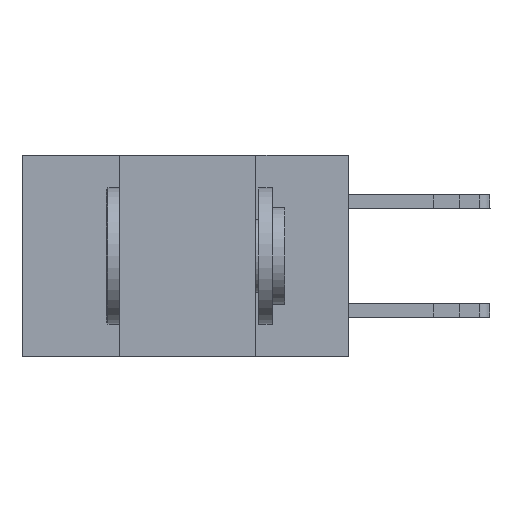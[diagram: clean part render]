
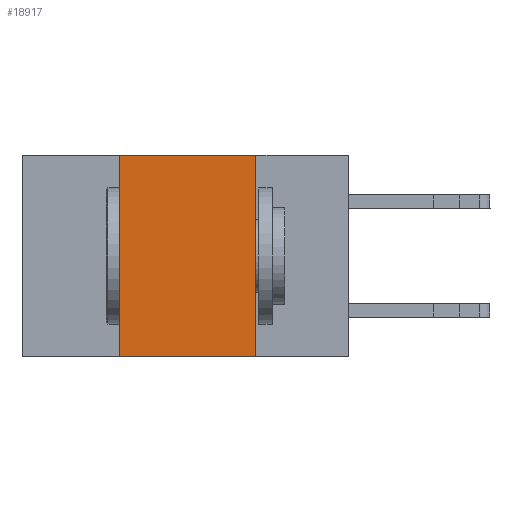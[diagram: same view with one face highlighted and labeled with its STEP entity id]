
A CAD part, left-side view. The second image highlights one B-rep face of the part: STEP entity #18917.
In plain terms, the highlighted planar face has unit normal (-1, 0, 0).
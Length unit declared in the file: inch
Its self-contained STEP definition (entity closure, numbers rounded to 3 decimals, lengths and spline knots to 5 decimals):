
#611 = VECTOR ( 'NONE', #9977, 39.37008 ) ;
#994 = CARTESIAN_POINT ( 'NONE',  ( 0., 0.6, -0.37 ) ) ;
#1306 = VERTEX_POINT ( 'NONE', #4158 ) ;
#1630 = LINE ( 'NONE', #3708, #611 ) ;
#2976 = CARTESIAN_POINT ( 'NONE',  ( 0., 0.6, 0. ) ) ;
#3246 = EDGE_CURVE ( 'NONE', #7535, #1306, #10115, .T. ) ;
#3393 = LINE ( 'NONE', #994, #19574 ) ;
#3580 = LINE ( 'NONE', #19640, #7327 ) ;
#3708 = CARTESIAN_POINT ( 'NONE',  ( 0., 0.42, 0. ) ) ;
#4158 = CARTESIAN_POINT ( 'NONE',  ( 0., 0.17, -0.37 ) ) ;
#6255 = EDGE_CURVE ( 'NONE', #6481, #7535, #3580, .T. ) ;
#6481 = VERTEX_POINT ( 'NONE', #8043 ) ;
#6937 = ORIENTED_EDGE ( 'NONE', *, *, #17049, .F. ) ;
#6992 = ORIENTED_EDGE ( 'NONE', *, *, #6255, .F. ) ;
#7317 = ORIENTED_EDGE ( 'NONE', *, *, #3246, .F. ) ;
#7327 = VECTOR ( 'NONE', #18459, 39.37008 ) ;
#7535 = VERTEX_POINT ( 'NONE', #12969 ) ;
#8043 = CARTESIAN_POINT ( 'NONE',  ( 0., 0.42, 0. ) ) ;
#8853 = VERTEX_POINT ( 'NONE', #11108 ) ;
#9977 = DIRECTION ( 'NONE',  ( 0., 0., 1. ) ) ;
#10115 = LINE ( 'NONE', #10811, #13798 ) ;
#10811 = CARTESIAN_POINT ( 'NONE',  ( 0., 0.17, 0. ) ) ;
#10896 = DIRECTION ( 'NONE',  ( 0., 0., -1. ) ) ;
#11091 = DIRECTION ( 'NONE',  ( 0., 0., -1. ) ) ;
#11108 = CARTESIAN_POINT ( 'NONE',  ( 0., 0.42, -0.37 ) ) ;
#12871 = ORIENTED_EDGE ( 'NONE', *, *, #16007, .T. ) ;
#12884 = FACE_OUTER_BOUND ( 'NONE', #17932, .T. ) ;
#12969 = CARTESIAN_POINT ( 'NONE',  ( 0., 0.17, 0. ) ) ;
#13798 = VECTOR ( 'NONE', #11091, 39.37008 ) ;
#15175 = DIRECTION ( 'NONE',  ( 0., -1., 0. ) ) ;
#15527 = PLANE ( 'NONE',  #17475 ) ;
#16007 = EDGE_CURVE ( 'NONE', #8853, #1306, #3393, .T. ) ;
#17049 = EDGE_CURVE ( 'NONE', #8853, #6481, #1630, .T. ) ;
#17475 = AXIS2_PLACEMENT_3D ( 'NONE', #2976, #20244, #10896 ) ;
#17932 = EDGE_LOOP ( 'NONE', ( #7317, #6992, #6937, #12871 ) ) ;
#18459 = DIRECTION ( 'NONE',  ( 0., -1., 0. ) ) ;
#18917 = ADVANCED_FACE ( 'NONE', ( #12884 ), #15527, .F. ) ;
#19574 = VECTOR ( 'NONE', #15175, 39.37008 ) ;
#19640 = CARTESIAN_POINT ( 'NONE',  ( 0., 0.6, 0. ) ) ;
#20244 = DIRECTION ( 'NONE',  ( 1., 0., 0. ) ) ;
